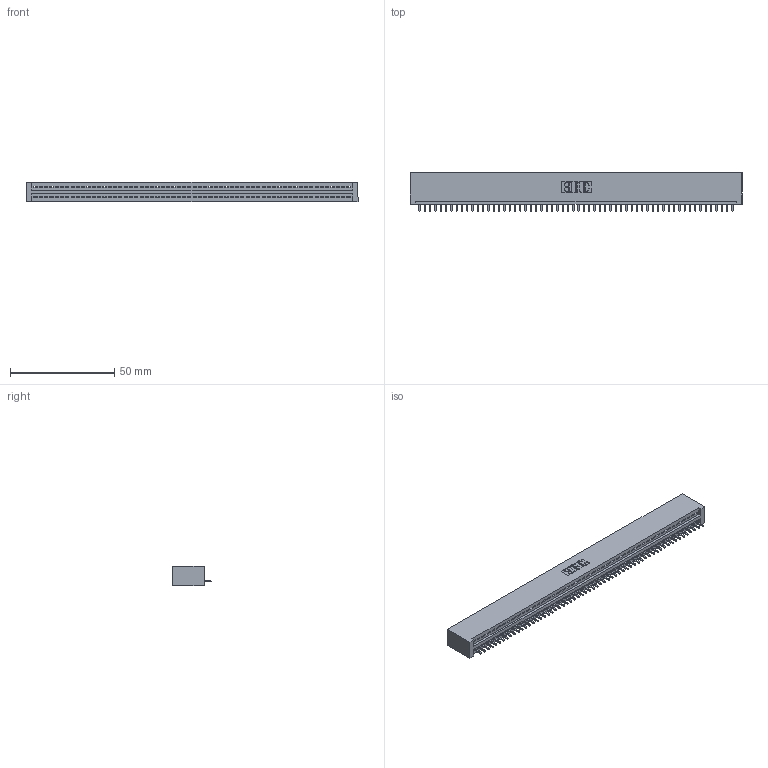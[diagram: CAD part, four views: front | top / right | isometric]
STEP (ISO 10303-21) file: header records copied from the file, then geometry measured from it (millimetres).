
FILE_DESCRIPTION (( 'STEP AP203' ), '1' );
FILE_NAME ('395-060-521-101.STEP', '2018-11-23T11:05:01', ( '' ), ( '' ), 'SwSTEP 2.0', 'SolidWorks 2016', '' );
FILE_SCHEMA (( 'CONFIG_CONTROL_DESIGN' ));
Length unit declared in the file: inch
Products named in the file (3): 395-060-521-101; 345-292-001_345-293-121; 345 Part_No Mounting Lugs
Assembly tree (61 placements, depth 2):
  395-060-521-101
    345 Part_No Mounting Lugs
    345-292-001_345-293-121  x60
Bounding box: 159 x 18.72 x 9.4 mm (x, y, z)
Volume: 15663.5 mm3; surface area: 20582.5 mm2
Topology: 61 solids, 61 shells, 3598 faces, 10877 edges, 7170 vertices
Faces by surface type: plane 2476, cylinder 1122
Entity records: 42475 total; most frequent: CARTESIAN_POINT 7364, ORIENTED_EDGE 7358, DIRECTION 6399, EDGE_CURVE 3679, LINE 3315, VECTOR 3315, VERTEX_POINT 2450, AXIS2_PLACEMENT_3D 1542
